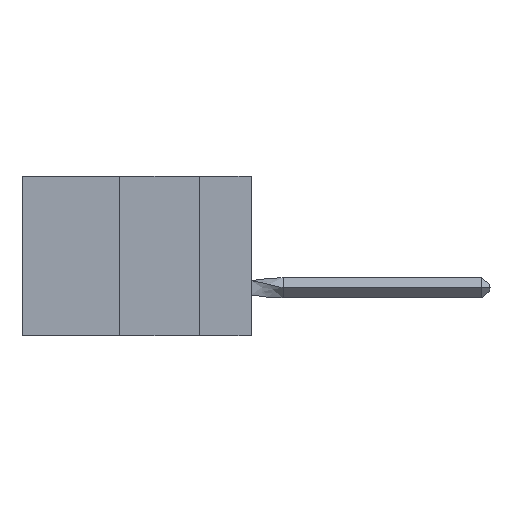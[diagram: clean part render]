
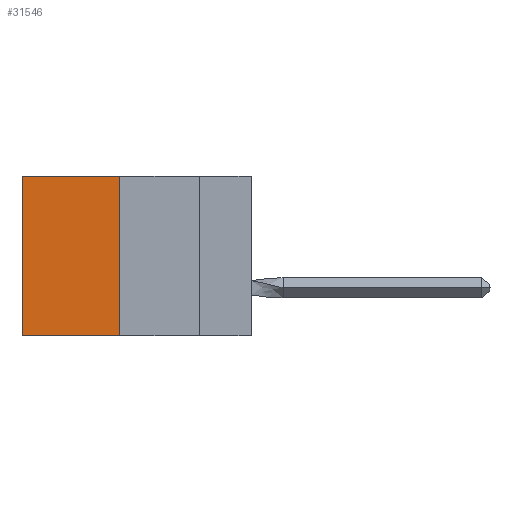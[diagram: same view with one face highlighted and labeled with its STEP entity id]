
A CAD part, left-side view. The second image highlights one B-rep face of the part: STEP entity #31546.
In plain terms, the highlighted planar face has unit normal (-1, 0, 0).
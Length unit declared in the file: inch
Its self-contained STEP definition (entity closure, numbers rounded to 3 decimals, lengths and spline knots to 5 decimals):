
#393 = AXIS2_PLACEMENT_3D ( 'NONE', #33696, #25431, #36566 ) ;
#571 = DIRECTION ( 'NONE',  ( 0., 1., 0. ) ) ;
#2383 = VECTOR ( 'NONE', #571, 39.37008 ) ;
#4569 = EDGE_LOOP ( 'NONE', ( #16695, #6623, #15377, #35270 ) ) ;
#5493 = LINE ( 'NONE', #7972, #11742 ) ;
#6623 = ORIENTED_EDGE ( 'NONE', *, *, #29382, .F. ) ;
#7972 = CARTESIAN_POINT ( 'NONE',  ( 0.305, 0.413, 0. ) ) ;
#9262 = VERTEX_POINT ( 'NONE', #26128 ) ;
#9944 = EDGE_CURVE ( 'NONE', #9262, #21978, #5493, .T. ) ;
#11361 = VECTOR ( 'NONE', #25368, 39.37008 ) ;
#11431 = LINE ( 'NONE', #13768, #21575 ) ;
#11742 = VECTOR ( 'NONE', #36234, 39.37008 ) ;
#13768 = CARTESIAN_POINT ( 'NONE',  ( 0.305, 0.72, -0.5 ) ) ;
#14755 = CARTESIAN_POINT ( 'NONE',  ( 0.305, 0.72, -0.5 ) ) ;
#14848 = LINE ( 'NONE', #36623, #11361 ) ;
#15377 = ORIENTED_EDGE ( 'NONE', *, *, #34408, .F. ) ;
#16695 = ORIENTED_EDGE ( 'NONE', *, *, #17551, .T. ) ;
#17551 = EDGE_CURVE ( 'NONE', #21978, #34861, #11431, .T. ) ;
#21575 = VECTOR ( 'NONE', #36124, 39.37008 ) ;
#21978 = VERTEX_POINT ( 'NONE', #32588 ) ;
#22463 = PLANE ( 'NONE',  #393 ) ;
#25368 = DIRECTION ( 'NONE',  ( 0., 0., -1. ) ) ;
#25431 = DIRECTION ( 'NONE',  ( 1., 0., 0. ) ) ;
#25587 = CARTESIAN_POINT ( 'NONE',  ( 0.305, 0.413, -0.5 ) ) ;
#26128 = CARTESIAN_POINT ( 'NONE',  ( 0.305, 0.413, 0. ) ) ;
#26744 = LINE ( 'NONE', #25587, #2383 ) ;
#27747 = CARTESIAN_POINT ( 'NONE',  ( 0.305, 0.413, -0.5 ) ) ;
#29382 = EDGE_CURVE ( 'NONE', #30192, #34861, #26744, .T. ) ;
#30192 = VERTEX_POINT ( 'NONE', #27747 ) ;
#31546 = ADVANCED_FACE ( 'NONE', ( #33095 ), #22463, .F. ) ;
#32588 = CARTESIAN_POINT ( 'NONE',  ( 0.305, 0.72, 0. ) ) ;
#33095 = FACE_OUTER_BOUND ( 'NONE', #4569, .T. ) ;
#33696 = CARTESIAN_POINT ( 'NONE',  ( 0.305, 0.413, -0.5 ) ) ;
#34408 = EDGE_CURVE ( 'NONE', #9262, #30192, #14848, .T. ) ;
#34861 = VERTEX_POINT ( 'NONE', #14755 ) ;
#35270 = ORIENTED_EDGE ( 'NONE', *, *, #9944, .T. ) ;
#36124 = DIRECTION ( 'NONE',  ( 0., 0., -1. ) ) ;
#36234 = DIRECTION ( 'NONE',  ( 0., 1., 0. ) ) ;
#36566 = DIRECTION ( 'NONE',  ( 0., 0., -1. ) ) ;
#36623 = CARTESIAN_POINT ( 'NONE',  ( 0.305, 0.413, -0.5 ) ) ;
